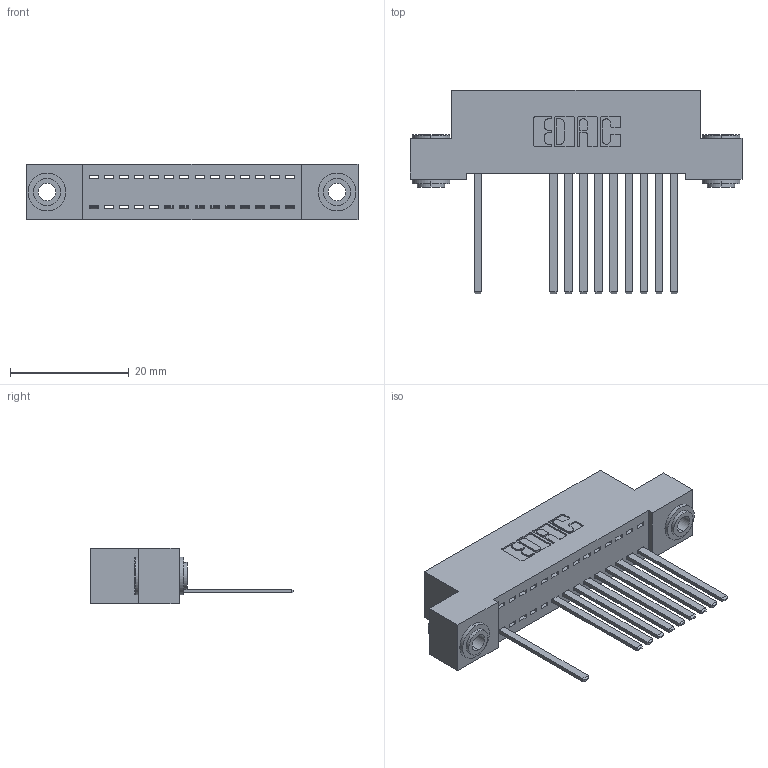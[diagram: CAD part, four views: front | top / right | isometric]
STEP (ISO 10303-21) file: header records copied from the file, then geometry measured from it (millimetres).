
FILE_DESCRIPTION (( 'STEP AP203' ), '1' );
FILE_NAME ('392-014-544-103.STEP', '2018-08-15T00:10:40', ( '' ), ( '' ), 'SwSTEP 2.0', 'SolidWorks 2016', '' );
FILE_SCHEMA (( 'CONFIG_CONTROL_DESIGN' ));
Length unit declared in the file: inch
Products named in the file (4): 345-292-001_345-293-144; 342-250-002_345-250-002-102; 392-014-544-103; 342 Part_.156 TH
Assembly tree (13 placements, depth 2):
  392-014-544-103
    342 Part_.156 TH
    345-292-001_345-293-144  x10
    342-250-002_345-250-002-102  x2
Bounding box: 55.88 x 34.3 x 9.4 mm (x, y, z)
Volume: 4889.3 mm3; surface area: 6975.7 mm2
Topology: 13 solids, 13 shells, 716 faces, 2123 edges, 1398 vertices
Faces by surface type: plane 504, cylinder 204, cone 8
Entity records: 12386 total; most frequent: CARTESIAN_POINT 2135, ORIENTED_EDGE 2082, DIRECTION 1883, EDGE_CURVE 1041, VECTOR 893, LINE 893, VERTEX_POINT 690, AXIS2_PLACEMENT_3D 495
